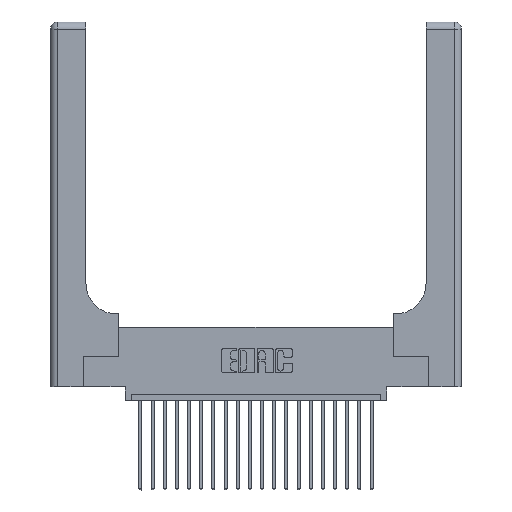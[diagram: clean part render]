
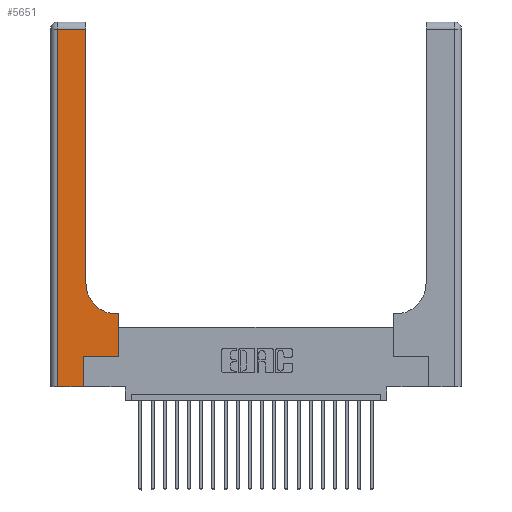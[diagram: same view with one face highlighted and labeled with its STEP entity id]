
A CAD part, top view. The second image highlights one B-rep face of the part: STEP entity #5651.
In plain terms, the highlighted planar face has unit normal (0, 0, 1).
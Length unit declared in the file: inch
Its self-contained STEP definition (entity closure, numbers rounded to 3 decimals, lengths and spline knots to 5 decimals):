
#428 = VECTOR ( 'NONE', #19657, 39.37008 ) ;
#1254 = DIRECTION ( 'NONE',  ( 1., 0., 0. ) ) ;
#1408 = VERTEX_POINT ( 'NONE', #1762 ) ;
#1481 = VECTOR ( 'NONE', #19652, 39.37008 ) ;
#1762 = CARTESIAN_POINT ( 'NONE',  ( 0.269, 0.25, 0.37 ) ) ;
#1952 = CARTESIAN_POINT ( 'NONE',  ( 0.5585, 0.25, 0.37 ) ) ;
#2368 = LINE ( 'NONE', #22566, #1481 ) ;
#3246 = CARTESIAN_POINT ( 'NONE',  ( 0.269, 0., 0.37 ) ) ;
#3292 = LINE ( 'NONE', #20716, #19385 ) ;
#3329 = EDGE_CURVE ( 'NONE', #16936, #22525, #3292, .T. ) ;
#3331 = CARTESIAN_POINT ( 'NONE',  ( 0.5415, 0.6, 0.37 ) ) ;
#3683 = ORIENTED_EDGE ( 'NONE', *, *, #13508, .T. ) ;
#4888 = CARTESIAN_POINT ( 'NONE',  ( 0.269, 0.25, 0.37 ) ) ;
#4900 = LINE ( 'NONE', #12574, #8324 ) ;
#5651 = ADVANCED_FACE ( 'NONE', ( #21251 ), #15098, .F. ) ;
#5723 = CARTESIAN_POINT ( 'NONE',  ( 0.269, 0., 0.37 ) ) ;
#5779 = DIRECTION ( 'NONE',  ( 0., -1., 0. ) ) ;
#6204 = VERTEX_POINT ( 'NONE', #1952 ) ;
#6238 = VERTEX_POINT ( 'NONE', #16836 ) ;
#7403 = ORIENTED_EDGE ( 'NONE', *, *, #8724, .T. ) ;
#8324 = VECTOR ( 'NONE', #13966, 39.37008 ) ;
#8463 = DIRECTION ( 'NONE',  ( 0., 1., 0. ) ) ;
#8724 = EDGE_CURVE ( 'NONE', #1408, #6204, #19523, .T. ) ;
#9175 = ORIENTED_EDGE ( 'NONE', *, *, #18683, .T. ) ;
#9502 = VERTEX_POINT ( 'NONE', #5723 ) ;
#10166 = LINE ( 'NONE', #3246, #10730 ) ;
#10423 = EDGE_CURVE ( 'NONE', #6238, #23204, #15252, .T. ) ;
#10552 = EDGE_CURVE ( 'NONE', #22525, #21187, #17501, .T. ) ;
#10725 = ORIENTED_EDGE ( 'NONE', *, *, #12959, .T. ) ;
#10730 = VECTOR ( 'NONE', #8463, 39.37008 ) ;
#10791 = CARTESIAN_POINT ( 'NONE',  ( 0., 2.94, 0.37 ) ) ;
#11039 = VECTOR ( 'NONE', #5779, 39.37008 ) ;
#11079 = EDGE_CURVE ( 'NONE', #9502, #1408, #10166, .T. ) ;
#11787 = CARTESIAN_POINT ( 'NONE',  ( 0., 3., 0.37 ) ) ;
#12574 = CARTESIAN_POINT ( 'NONE',  ( 0.2915, 3., 0.37 ) ) ;
#12959 = EDGE_CURVE ( 'NONE', #20164, #6238, #15123, .T. ) ;
#13310 = ORIENTED_EDGE ( 'NONE', *, *, #3329, .T. ) ;
#13473 = DIRECTION ( 'NONE',  ( 1., 0., 0. ) ) ;
#13508 = EDGE_CURVE ( 'NONE', #21187, #20164, #4900, .T. ) ;
#13966 = DIRECTION ( 'NONE',  ( 0., 1., 0. ) ) ;
#14044 = ORIENTED_EDGE ( 'NONE', *, *, #10423, .T. ) ;
#14836 = EDGE_LOOP ( 'NONE', ( #3683, #10725, #14044, #21700, #20795, #7403, #9175, #13310, #17700 ) ) ;
#14917 = CARTESIAN_POINT ( 'NONE',  ( 0.06, 3., 0.37 ) ) ;
#15098 = PLANE ( 'NONE',  #17187 ) ;
#15123 = LINE ( 'NONE', #10791, #428 ) ;
#15252 = LINE ( 'NONE', #14917, #11039 ) ;
#15537 = CARTESIAN_POINT ( 'NONE',  ( 0.2915, 2.94, 0.37 ) ) ;
#16836 = CARTESIAN_POINT ( 'NONE',  ( 0.06, 2.94, 0.37 ) ) ;
#16936 = VERTEX_POINT ( 'NONE', #22945 ) ;
#17187 = AXIS2_PLACEMENT_3D ( 'NONE', #11787, #20542, #18853 ) ;
#17501 = CIRCLE ( 'NONE', #19063, 0.25 ) ;
#17700 = ORIENTED_EDGE ( 'NONE', *, *, #10552, .T. ) ;
#17748 = CARTESIAN_POINT ( 'NONE',  ( 0.2915, 0.85, 0.37 ) ) ;
#17929 = LINE ( 'NONE', #23348, #19052 ) ;
#18683 = EDGE_CURVE ( 'NONE', #6204, #16936, #17929, .T. ) ;
#18741 = CARTESIAN_POINT ( 'NONE',  ( 0.5415, 0.85, 0.37 ) ) ;
#18853 = DIRECTION ( 'NONE',  ( -1., 0., 0. ) ) ;
#19052 = VECTOR ( 'NONE', #21232, 39.37008 ) ;
#19063 = AXIS2_PLACEMENT_3D ( 'NONE', #18741, #22384, #13473 ) ;
#19385 = VECTOR ( 'NONE', #22370, 39.37008 ) ;
#19523 = LINE ( 'NONE', #4888, #23198 ) ;
#19602 = CARTESIAN_POINT ( 'NONE',  ( 0.06, 0., 0.37 ) ) ;
#19610 = EDGE_CURVE ( 'NONE', #23204, #9502, #2368, .T. ) ;
#19652 = DIRECTION ( 'NONE',  ( 1., 0., 0. ) ) ;
#19657 = DIRECTION ( 'NONE',  ( -1., 0., 0. ) ) ;
#20164 = VERTEX_POINT ( 'NONE', #15537 ) ;
#20542 = DIRECTION ( 'NONE',  ( 0., 0., -1. ) ) ;
#20716 = CARTESIAN_POINT ( 'NONE',  ( 0.2915, 0.6, 0.37 ) ) ;
#20795 = ORIENTED_EDGE ( 'NONE', *, *, #11079, .T. ) ;
#21187 = VERTEX_POINT ( 'NONE', #17748 ) ;
#21232 = DIRECTION ( 'NONE',  ( 0., 1., 0. ) ) ;
#21251 = FACE_OUTER_BOUND ( 'NONE', #14836, .T. ) ;
#21700 = ORIENTED_EDGE ( 'NONE', *, *, #19610, .T. ) ;
#22370 = DIRECTION ( 'NONE',  ( -1., 0., 0. ) ) ;
#22384 = DIRECTION ( 'NONE',  ( 0., 0., -1. ) ) ;
#22525 = VERTEX_POINT ( 'NONE', #3331 ) ;
#22566 = CARTESIAN_POINT ( 'NONE',  ( 0., 0., 0.37 ) ) ;
#22945 = CARTESIAN_POINT ( 'NONE',  ( 0.5585, 0.6, 0.37 ) ) ;
#23198 = VECTOR ( 'NONE', #1254, 39.37008 ) ;
#23204 = VERTEX_POINT ( 'NONE', #19602 ) ;
#23348 = CARTESIAN_POINT ( 'NONE',  ( 0.5585, 0.25, 0.37 ) ) ;
